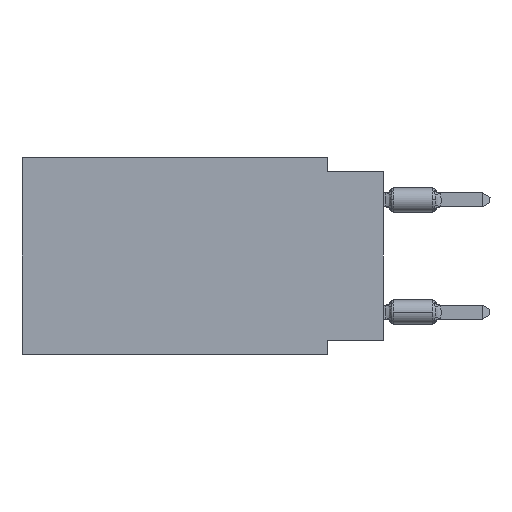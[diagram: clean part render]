
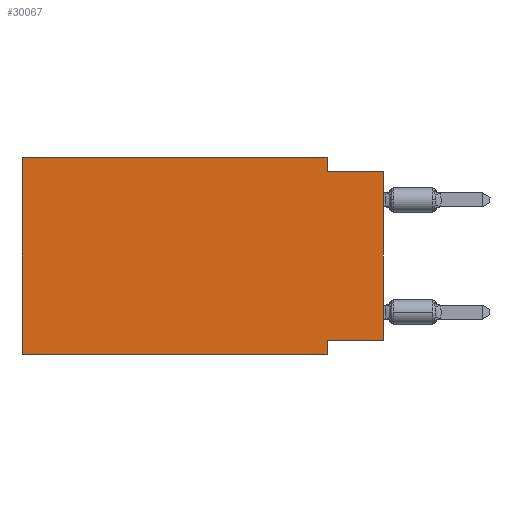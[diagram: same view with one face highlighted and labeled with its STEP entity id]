
A CAD part, left-side view. The second image highlights one B-rep face of the part: STEP entity #30067.
In plain terms, the highlighted planar face has unit normal (-1, 0, 0).
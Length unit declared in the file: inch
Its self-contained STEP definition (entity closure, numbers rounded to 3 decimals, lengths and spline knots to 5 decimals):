
#664 = ORIENTED_EDGE ( 'NONE', *, *, #12845, .F. ) ;
#2439 = VERTEX_POINT ( 'NONE', #5039 ) ;
#4805 = ORIENTED_EDGE ( 'NONE', *, *, #21589, .F. ) ;
#4935 = ORIENTED_EDGE ( 'NONE', *, *, #25550, .F. ) ;
#5039 = CARTESIAN_POINT ( 'NONE',  ( 0., 0.1, -0.35 ) ) ;
#5717 = DIRECTION ( 'NONE',  ( 0., 1., 0. ) ) ;
#5969 = VERTEX_POINT ( 'NONE', #40500 ) ;
#6566 = LINE ( 'NONE', #23677, #45086 ) ;
#6615 = VECTOR ( 'NONE', #53544, 39.37008 ) ;
#6932 = CARTESIAN_POINT ( 'NONE',  ( 0., 0., -0.325 ) ) ;
#7256 = DIRECTION ( 'NONE',  ( 0., 0., -1. ) ) ;
#10802 = FACE_OUTER_BOUND ( 'NONE', #32484, .T. ) ;
#11289 = CARTESIAN_POINT ( 'NONE',  ( 0., 0., -0.325 ) ) ;
#12493 = EDGE_CURVE ( 'NONE', #5969, #2439, #41180, .T. ) ;
#12845 = EDGE_CURVE ( 'NONE', #5969, #15890, #25838, .T. ) ;
#15040 = VERTEX_POINT ( 'NONE', #31828 ) ;
#15890 = VERTEX_POINT ( 'NONE', #26833 ) ;
#16312 = EDGE_CURVE ( 'NONE', #55993, #15040, #17655, .T. ) ;
#17655 = LINE ( 'NONE', #35573, #6615 ) ;
#20120 = AXIS2_PLACEMENT_3D ( 'NONE', #20798, #42874, #7256 ) ;
#20798 = CARTESIAN_POINT ( 'NONE',  ( 0., 0.645, 0. ) ) ;
#21589 = EDGE_CURVE ( 'NONE', #47531, #2439, #57944, .T. ) ;
#21743 = DIRECTION ( 'NONE',  ( 0., 0., -1. ) ) ;
#22211 = VECTOR ( 'NONE', #55480, 39.37008 ) ;
#23266 = ORIENTED_EDGE ( 'NONE', *, *, #16312, .T. ) ;
#23527 = CARTESIAN_POINT ( 'NONE',  ( 0., 0.645, -0.35 ) ) ;
#23677 = CARTESIAN_POINT ( 'NONE',  ( 0., 0.1, 0. ) ) ;
#24285 = LINE ( 'NONE', #42229, #22211 ) ;
#24793 = VECTOR ( 'NONE', #21743, 39.37008 ) ;
#25550 = EDGE_CURVE ( 'NONE', #15890, #37850, #36927, .T. ) ;
#25675 = ORIENTED_EDGE ( 'NONE', *, *, #56415, .F. ) ;
#25838 = LINE ( 'NONE', #52906, #46003 ) ;
#26833 = CARTESIAN_POINT ( 'NONE',  ( 0., 0.645, 0. ) ) ;
#28501 = DIRECTION ( 'NONE',  ( 0., -1., 0. ) ) ;
#28644 = CARTESIAN_POINT ( 'NONE',  ( 0., 0.1, -0.325 ) ) ;
#28954 = CARTESIAN_POINT ( 'NONE',  ( 0., 0.645, 0. ) ) ;
#29064 = ORIENTED_EDGE ( 'NONE', *, *, #12493, .T. ) ;
#30067 = ADVANCED_FACE ( 'NONE', ( #10802 ), #51110, .F. ) ;
#31828 = CARTESIAN_POINT ( 'NONE',  ( 0., 0., -0.025 ) ) ;
#32196 = CARTESIAN_POINT ( 'NONE',  ( 0., 0.1, -0.025 ) ) ;
#32484 = EDGE_LOOP ( 'NONE', ( #23266, #51865, #33403, #4935, #664, #29064, #4805, #25675 ) ) ;
#33403 = ORIENTED_EDGE ( 'NONE', *, *, #56419, .F. ) ;
#35257 = CARTESIAN_POINT ( 'NONE',  ( 0., 0.1, -0.35 ) ) ;
#35573 = CARTESIAN_POINT ( 'NONE',  ( 0., 0., 0. ) ) ;
#36624 = VECTOR ( 'NONE', #5717, 39.37008 ) ;
#36927 = LINE ( 'NONE', #28954, #44936 ) ;
#37850 = VERTEX_POINT ( 'NONE', #54157 ) ;
#39822 = VERTEX_POINT ( 'NONE', #32196 ) ;
#40500 = CARTESIAN_POINT ( 'NONE',  ( 0., 0.645, -0.35 ) ) ;
#41180 = LINE ( 'NONE', #23527, #49759 ) ;
#41620 = DIRECTION ( 'NONE',  ( 0., 0., -1. ) ) ;
#42229 = CARTESIAN_POINT ( 'NONE',  ( 0., 0., -0.025 ) ) ;
#42874 = DIRECTION ( 'NONE',  ( 1., 0., 0. ) ) ;
#43799 = DIRECTION ( 'NONE',  ( 0., 0., 1. ) ) ;
#44936 = VECTOR ( 'NONE', #54893, 39.37008 ) ;
#45086 = VECTOR ( 'NONE', #41620, 39.37008 ) ;
#46003 = VECTOR ( 'NONE', #43799, 39.37008 ) ;
#46889 = LINE ( 'NONE', #11289, #36624 ) ;
#47531 = VERTEX_POINT ( 'NONE', #28644 ) ;
#49759 = VECTOR ( 'NONE', #28501, 39.37008 ) ;
#51110 = PLANE ( 'NONE',  #20120 ) ;
#51865 = ORIENTED_EDGE ( 'NONE', *, *, #57594, .F. ) ;
#52906 = CARTESIAN_POINT ( 'NONE',  ( 0., 0.645, 0. ) ) ;
#53544 = DIRECTION ( 'NONE',  ( 0., 0., 1. ) ) ;
#54157 = CARTESIAN_POINT ( 'NONE',  ( 0., 0.1, 0. ) ) ;
#54893 = DIRECTION ( 'NONE',  ( 0., -1., 0. ) ) ;
#55480 = DIRECTION ( 'NONE',  ( 0., -1., 0. ) ) ;
#55993 = VERTEX_POINT ( 'NONE', #6932 ) ;
#56415 = EDGE_CURVE ( 'NONE', #55993, #47531, #46889, .T. ) ;
#56419 = EDGE_CURVE ( 'NONE', #37850, #39822, #6566, .T. ) ;
#57594 = EDGE_CURVE ( 'NONE', #39822, #15040, #24285, .T. ) ;
#57944 = LINE ( 'NONE', #35257, #24793 ) ;
